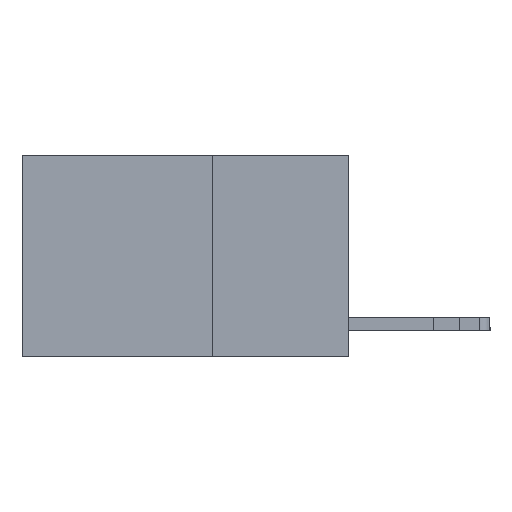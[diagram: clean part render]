
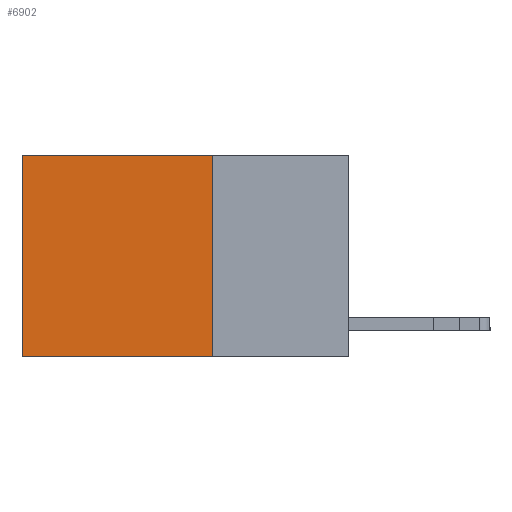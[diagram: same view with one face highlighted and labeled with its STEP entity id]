
A CAD part, left-side view. The second image highlights one B-rep face of the part: STEP entity #6902.
In plain terms, the highlighted planar face has unit normal (-1, 0, 0).
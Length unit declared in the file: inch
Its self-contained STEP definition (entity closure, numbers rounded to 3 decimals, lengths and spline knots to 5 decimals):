
#636 = LINE ( 'NONE', #7947, #3416 ) ;
#1467 = CARTESIAN_POINT ( 'NONE',  ( 0.2625, 0.25, 0. ) ) ;
#1879 = LINE ( 'NONE', #13499, #3185 ) ;
#2168 = VERTEX_POINT ( 'NONE', #2662 ) ;
#2662 = CARTESIAN_POINT ( 'NONE',  ( 0.2625, 0.6, 0. ) ) ;
#3006 = PLANE ( 'NONE',  #9561 ) ;
#3185 = VECTOR ( 'NONE', #9241, 39.37008 ) ;
#3273 = VERTEX_POINT ( 'NONE', #5037 ) ;
#3416 = VECTOR ( 'NONE', #4850, 39.37008 ) ;
#3720 = CARTESIAN_POINT ( 'NONE',  ( 0.2625, 0.25, 0. ) ) ;
#4111 = LINE ( 'NONE', #12547, #13275 ) ;
#4622 = LINE ( 'NONE', #3720, #5101 ) ;
#4850 = DIRECTION ( 'NONE',  ( 0., 0., -1. ) ) ;
#4933 = CARTESIAN_POINT ( 'NONE',  ( 0.2625, 0.25, 0. ) ) ;
#5037 = CARTESIAN_POINT ( 'NONE',  ( 0.2625, 0.6, -0.37 ) ) ;
#5101 = VECTOR ( 'NONE', #12030, 39.37008 ) ;
#5278 = EDGE_LOOP ( 'NONE', ( #9608, #12824, #10513, #7902 ) ) ;
#5965 = DIRECTION ( 'NONE',  ( 0., 0., -1. ) ) ;
#6902 = ADVANCED_FACE ( 'NONE', ( #9191 ), #3006, .F. ) ;
#7271 = DIRECTION ( 'NONE',  ( 1., 0., 0. ) ) ;
#7680 = CARTESIAN_POINT ( 'NONE',  ( 0.2625, 0.25, -0.37 ) ) ;
#7902 = ORIENTED_EDGE ( 'NONE', *, *, #12833, .T. ) ;
#7947 = CARTESIAN_POINT ( 'NONE',  ( 0.2625, 0.6, 0. ) ) ;
#8312 = DIRECTION ( 'NONE',  ( 0., 1., 0. ) ) ;
#8315 = EDGE_CURVE ( 'NONE', #9044, #3273, #4111, .T. ) ;
#9044 = VERTEX_POINT ( 'NONE', #7680 ) ;
#9191 = FACE_OUTER_BOUND ( 'NONE', #5278, .T. ) ;
#9241 = DIRECTION ( 'NONE',  ( 0., 0., -1. ) ) ;
#9561 = AXIS2_PLACEMENT_3D ( 'NONE', #4933, #7271, #5965 ) ;
#9608 = ORIENTED_EDGE ( 'NONE', *, *, #10762, .T. ) ;
#10513 = ORIENTED_EDGE ( 'NONE', *, *, #10850, .F. ) ;
#10762 = EDGE_CURVE ( 'NONE', #2168, #3273, #636, .T. ) ;
#10850 = EDGE_CURVE ( 'NONE', #12262, #9044, #1879, .T. ) ;
#12030 = DIRECTION ( 'NONE',  ( 0., 1., 0. ) ) ;
#12262 = VERTEX_POINT ( 'NONE', #1467 ) ;
#12547 = CARTESIAN_POINT ( 'NONE',  ( 0.2625, 0.25, -0.37 ) ) ;
#12824 = ORIENTED_EDGE ( 'NONE', *, *, #8315, .F. ) ;
#12833 = EDGE_CURVE ( 'NONE', #12262, #2168, #4622, .T. ) ;
#13275 = VECTOR ( 'NONE', #8312, 39.37008 ) ;
#13499 = CARTESIAN_POINT ( 'NONE',  ( 0.2625, 0.25, 0. ) ) ;
